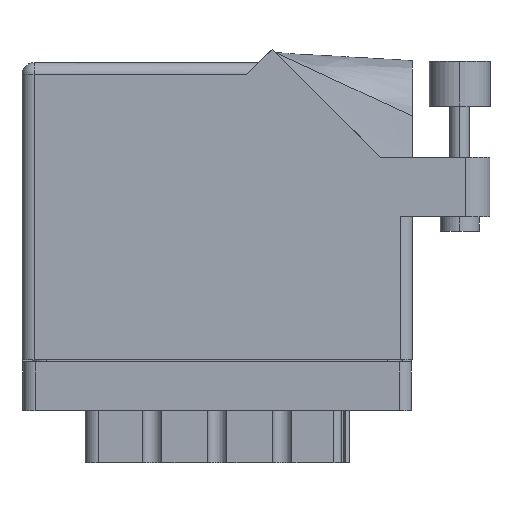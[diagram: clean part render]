
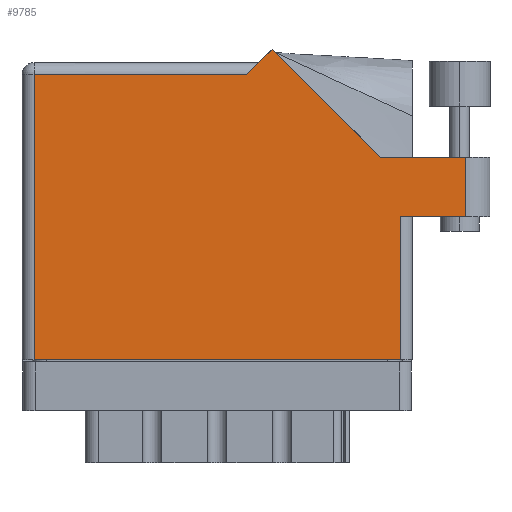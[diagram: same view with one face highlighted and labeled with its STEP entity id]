
A CAD part, front view. The second image highlights one B-rep face of the part: STEP entity #9785.
In plain terms, the highlighted face is planar.
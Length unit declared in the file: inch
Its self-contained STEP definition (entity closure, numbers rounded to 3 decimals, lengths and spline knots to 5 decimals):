
#1858 = CARTESIAN_POINT ( 'NONE',  ( 1.28771, 1.60071, 0. ) ) ;
#1872 = DIRECTION ( 'NONE',  ( 0., 0., -1. ) ) ;
#1900 = ORIENTED_EDGE ( 'NONE', *, *, #28600, .T. ) ;
#2143 = VERTEX_POINT ( 'NONE', #24574 ) ;
#3253 = EDGE_CURVE ( 'NONE', #12386, #13843, #29176, .T. ) ;
#4900 = VECTOR ( 'NONE', #31173, 39.37008 ) ;
#5614 = VERTEX_POINT ( 'NONE', #1858 ) ;
#5686 = VECTOR ( 'NONE', #36413, 39.37008 ) ;
#6251 = VERTEX_POINT ( 'NONE', #26975 ) ;
#6870 = DIRECTION ( 'NONE',  ( -0.707, 0.707, 0. ) ) ;
#7164 = DIRECTION ( 'NONE',  ( -1., 0., 0. ) ) ;
#7227 = CARTESIAN_POINT ( 'NONE',  ( 1.84442, 1.044, 0. ) ) ;
#7648 = LINE ( 'NONE', #11014, #31891 ) ;
#8164 = CARTESIAN_POINT ( 'NONE',  ( 2.285, 1.044, 0. ) ) ;
#8791 = CARTESIAN_POINT ( 'NONE',  ( 2.01, 0.737, 0. ) ) ;
#9466 = ORIENTED_EDGE ( 'NONE', *, *, #17659, .T. ) ;
#9785 = ADVANCED_FACE ( 'NONE', ( #10341 ), #21831, .F. ) ;
#9975 = CARTESIAN_POINT ( 'NONE',  ( 0., 1.53, 0. ) ) ;
#10341 = FACE_OUTER_BOUND ( 'NONE', #18183, .T. ) ;
#10377 = ORIENTED_EDGE ( 'NONE', *, *, #36051, .T. ) ;
#10818 = CARTESIAN_POINT ( 'NONE',  ( 1.948, 0.737, 0. ) ) ;
#11014 = CARTESIAN_POINT ( 'NONE',  ( 0.062, 0., 0. ) ) ;
#11887 = EDGE_CURVE ( 'NONE', #34112, #6251, #20028, .T. ) ;
#12204 = CARTESIAN_POINT ( 'NONE',  ( 1.948, 0., 0. ) ) ;
#12386 = VERTEX_POINT ( 'NONE', #8164 ) ;
#13843 = VERTEX_POINT ( 'NONE', #19030 ) ;
#14555 = CARTESIAN_POINT ( 'NONE',  ( 1.217, 1.53, 0. ) ) ;
#16332 = VECTOR ( 'NONE', #6870, 39.37008 ) ;
#17659 = EDGE_CURVE ( 'NONE', #20701, #12386, #30702, .T. ) ;
#18183 = EDGE_LOOP ( 'NONE', ( #27646, #9466, #24700, #1900, #32233, #23192, #10377, #26189, #34251 ) ) ;
#18333 = LINE ( 'NONE', #7227, #16332 ) ;
#18748 = EDGE_CURVE ( 'NONE', #6251, #20701, #29098, .T. ) ;
#18938 = VECTOR ( 'NONE', #23440, 39.37008 ) ;
#19030 = CARTESIAN_POINT ( 'NONE',  ( 1.84442, 1.044, 0. ) ) ;
#19759 = CARTESIAN_POINT ( 'NONE',  ( 1.155, 1.468, 0. ) ) ;
#19783 = CARTESIAN_POINT ( 'NONE',  ( 2.41, 1.044, 0. ) ) ;
#20028 = LINE ( 'NONE', #10818, #5686 ) ;
#20153 = VECTOR ( 'NONE', #26332, 39.37008 ) ;
#20293 = VECTOR ( 'NONE', #33360, 39.37008 ) ;
#20701 = VERTEX_POINT ( 'NONE', #29307 ) ;
#21831 = PLANE ( 'NONE',  #35451 ) ;
#21982 = CARTESIAN_POINT ( 'NONE',  ( 0., 1.468, 0. ) ) ;
#22162 = LINE ( 'NONE', #21982, #4900 ) ;
#22485 = LINE ( 'NONE', #14555, #36171 ) ;
#23176 = CARTESIAN_POINT ( 'NONE',  ( 0.062, 0., 0. ) ) ;
#23192 = ORIENTED_EDGE ( 'NONE', *, *, #34365, .T. ) ;
#23440 = DIRECTION ( 'NONE',  ( 1., 0., 0. ) ) ;
#23598 = VERTEX_POINT ( 'NONE', #19759 ) ;
#24137 = EDGE_CURVE ( 'NONE', #34942, #34112, #26260, .T. ) ;
#24574 = CARTESIAN_POINT ( 'NONE',  ( 0.062, 1.468, 0. ) ) ;
#24700 = ORIENTED_EDGE ( 'NONE', *, *, #3253, .T. ) ;
#25478 = DIRECTION ( 'NONE',  ( -0.707, -0.707, 0. ) ) ;
#26189 = ORIENTED_EDGE ( 'NONE', *, *, #24137, .T. ) ;
#26260 = LINE ( 'NONE', #26442, #18938 ) ;
#26332 = DIRECTION ( 'NONE',  ( -1., 0., 0. ) ) ;
#26344 = VECTOR ( 'NONE', #26640, 39.37008 ) ;
#26442 = CARTESIAN_POINT ( 'NONE',  ( 0., 0., 0. ) ) ;
#26640 = DIRECTION ( 'NONE',  ( 1., 0., 0. ) ) ;
#26975 = CARTESIAN_POINT ( 'NONE',  ( 1.948, 0.737, 0. ) ) ;
#27646 = ORIENTED_EDGE ( 'NONE', *, *, #18748, .T. ) ;
#28600 = EDGE_CURVE ( 'NONE', #13843, #5614, #18333, .T. ) ;
#29098 = LINE ( 'NONE', #8791, #26344 ) ;
#29176 = LINE ( 'NONE', #19783, #20153 ) ;
#29307 = CARTESIAN_POINT ( 'NONE',  ( 2.285, 0.737, 0. ) ) ;
#30677 = EDGE_CURVE ( 'NONE', #5614, #23598, #22485, .T. ) ;
#30702 = LINE ( 'NONE', #36167, #20293 ) ;
#31173 = DIRECTION ( 'NONE',  ( -1., 0., 0. ) ) ;
#31891 = VECTOR ( 'NONE', #33594, 39.37008 ) ;
#32233 = ORIENTED_EDGE ( 'NONE', *, *, #30677, .T. ) ;
#33360 = DIRECTION ( 'NONE',  ( 0., 1., 0. ) ) ;
#33594 = DIRECTION ( 'NONE',  ( 0., -1., 0. ) ) ;
#34112 = VERTEX_POINT ( 'NONE', #12204 ) ;
#34251 = ORIENTED_EDGE ( 'NONE', *, *, #11887, .T. ) ;
#34365 = EDGE_CURVE ( 'NONE', #23598, #2143, #22162, .T. ) ;
#34942 = VERTEX_POINT ( 'NONE', #23176 ) ;
#35451 = AXIS2_PLACEMENT_3D ( 'NONE', #9975, #1872, #7164 ) ;
#36051 = EDGE_CURVE ( 'NONE', #2143, #34942, #7648, .T. ) ;
#36167 = CARTESIAN_POINT ( 'NONE',  ( 2.285, 1.044, 0. ) ) ;
#36171 = VECTOR ( 'NONE', #25478, 39.37008 ) ;
#36413 = DIRECTION ( 'NONE',  ( 0., 1., 0. ) ) ;
